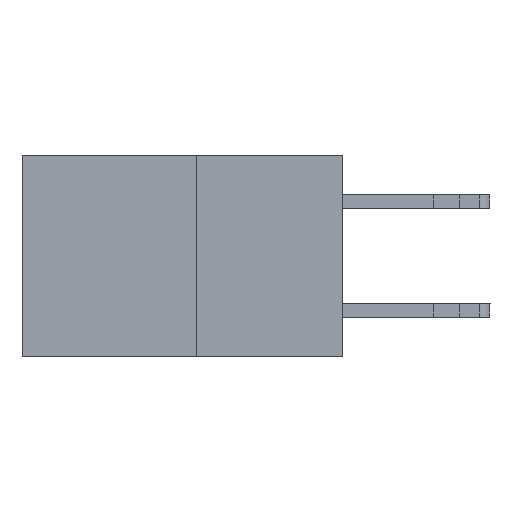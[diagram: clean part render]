
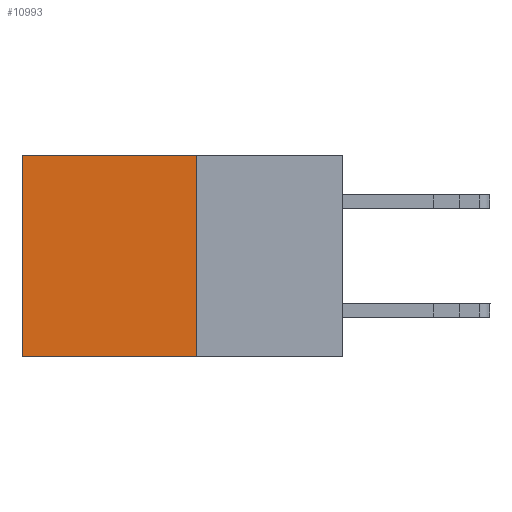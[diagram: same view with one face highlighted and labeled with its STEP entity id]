
A CAD part, left-side view. The second image highlights one B-rep face of the part: STEP entity #10993.
In plain terms, the highlighted planar face has unit normal (-1, 0, 0).
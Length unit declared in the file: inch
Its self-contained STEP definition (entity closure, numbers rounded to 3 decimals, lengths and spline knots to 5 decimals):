
#264 = FACE_OUTER_BOUND ( 'NONE', #4057, .T. ) ;
#541 = VECTOR ( 'NONE', #2147, 39.37008 ) ;
#1059 = EDGE_CURVE ( 'NONE', #13284, #11031, #17767, .T. ) ;
#1591 = ORIENTED_EDGE ( 'NONE', *, *, #17906, .F. ) ;
#1810 = CARTESIAN_POINT ( 'NONE',  ( 0.277, 0.27, -0.37 ) ) ;
#2147 = DIRECTION ( 'NONE',  ( 0., 1., 0. ) ) ;
#2600 = VERTEX_POINT ( 'NONE', #18485 ) ;
#3261 = DIRECTION ( 'NONE',  ( 0., 1., 0. ) ) ;
#4057 = EDGE_LOOP ( 'NONE', ( #5848, #1591, #4626, #13878 ) ) ;
#4626 = ORIENTED_EDGE ( 'NONE', *, *, #15026, .F. ) ;
#5740 = CARTESIAN_POINT ( 'NONE',  ( 0.277, 0.27, 0. ) ) ;
#5848 = ORIENTED_EDGE ( 'NONE', *, *, #9937, .T. ) ;
#6243 = DIRECTION ( 'NONE',  ( 0., 0., -1. ) ) ;
#6520 = AXIS2_PLACEMENT_3D ( 'NONE', #20847, #22805, #10929 ) ;
#6611 = VECTOR ( 'NONE', #6243, 39.37008 ) ;
#6899 = PLANE ( 'NONE',  #6520 ) ;
#7415 = CARTESIAN_POINT ( 'NONE',  ( 0.277, 0.27, -0.37 ) ) ;
#8834 = LINE ( 'NONE', #7415, #18808 ) ;
#9596 = CARTESIAN_POINT ( 'NONE',  ( 0.277, 0.27, 0. ) ) ;
#9937 = EDGE_CURVE ( 'NONE', #11031, #2600, #22481, .T. ) ;
#10929 = DIRECTION ( 'NONE',  ( 0., 0., -1. ) ) ;
#10993 = ADVANCED_FACE ( 'NONE', ( #264 ), #6899, .F. ) ;
#11031 = VERTEX_POINT ( 'NONE', #24882 ) ;
#12921 = CARTESIAN_POINT ( 'NONE',  ( 0.277, 0.59, -0.37 ) ) ;
#13223 = CARTESIAN_POINT ( 'NONE',  ( 0.277, 0.27, -0.37 ) ) ;
#13284 = VERTEX_POINT ( 'NONE', #9596 ) ;
#13878 = ORIENTED_EDGE ( 'NONE', *, *, #1059, .T. ) ;
#13896 = VECTOR ( 'NONE', #3261, 39.37008 ) ;
#14532 = LINE ( 'NONE', #13223, #13896 ) ;
#15026 = EDGE_CURVE ( 'NONE', #13284, #21381, #8834, .T. ) ;
#17767 = LINE ( 'NONE', #5740, #541 ) ;
#17906 = EDGE_CURVE ( 'NONE', #21381, #2600, #14532, .T. ) ;
#18485 = CARTESIAN_POINT ( 'NONE',  ( 0.277, 0.59, -0.37 ) ) ;
#18808 = VECTOR ( 'NONE', #19339, 39.37008 ) ;
#19339 = DIRECTION ( 'NONE',  ( 0., 0., -1. ) ) ;
#20847 = CARTESIAN_POINT ( 'NONE',  ( 0.277, 0.27, -0.37 ) ) ;
#21381 = VERTEX_POINT ( 'NONE', #1810 ) ;
#22481 = LINE ( 'NONE', #12921, #6611 ) ;
#22805 = DIRECTION ( 'NONE',  ( 1., 0., 0. ) ) ;
#24882 = CARTESIAN_POINT ( 'NONE',  ( 0.277, 0.59, 0. ) ) ;
